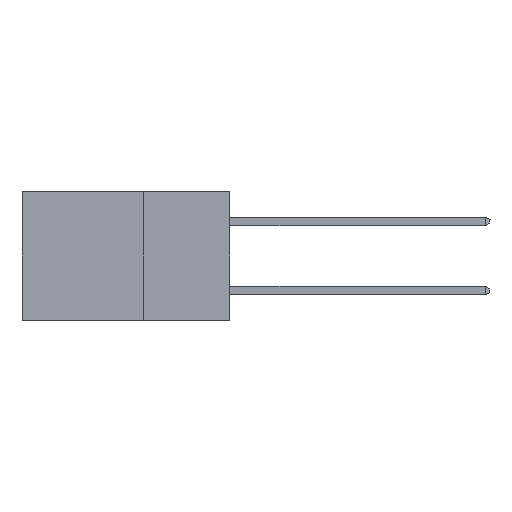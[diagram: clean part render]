
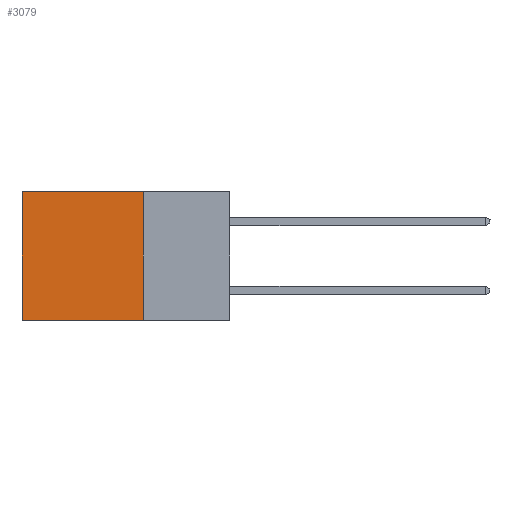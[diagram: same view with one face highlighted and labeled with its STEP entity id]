
A CAD part, left-side view. The second image highlights one B-rep face of the part: STEP entity #3079.
In plain terms, the highlighted planar face has unit normal (-1, 0, 0).
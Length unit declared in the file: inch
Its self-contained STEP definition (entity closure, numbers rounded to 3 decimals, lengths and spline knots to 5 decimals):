
#244 = DIRECTION ( 'NONE',  ( 0., 1., 0. ) ) ;
#1169 = ORIENTED_EDGE ( 'NONE', *, *, #16890, .F. ) ;
#1920 = VECTOR ( 'NONE', #7030, 39.37008 ) ;
#2679 = ORIENTED_EDGE ( 'NONE', *, *, #18009, .T. ) ;
#3079 = ADVANCED_FACE ( 'NONE', ( #25911 ), #11441, .F. ) ;
#3722 = CARTESIAN_POINT ( 'NONE',  ( 0.298, 0.6, -0.37 ) ) ;
#4624 = CARTESIAN_POINT ( 'NONE',  ( 0.298, 0.6, 0. ) ) ;
#5027 = CARTESIAN_POINT ( 'NONE',  ( 0.298, 0.25, 0. ) ) ;
#6023 = DIRECTION ( 'NONE',  ( 0., 0., -1. ) ) ;
#6082 = EDGE_CURVE ( 'NONE', #16232, #9276, #14364, .T. ) ;
#6126 = LINE ( 'NONE', #19397, #12522 ) ;
#6739 = CARTESIAN_POINT ( 'NONE',  ( 0.298, 0.25, 0. ) ) ;
#6807 = CARTESIAN_POINT ( 'NONE',  ( 0.298, 0.25, 0. ) ) ;
#6871 = CARTESIAN_POINT ( 'NONE',  ( 0.298, 0.6, 0. ) ) ;
#7030 = DIRECTION ( 'NONE',  ( 0., 0., -1. ) ) ;
#9276 = VERTEX_POINT ( 'NONE', #6871 ) ;
#9402 = VECTOR ( 'NONE', #6023, 39.37008 ) ;
#11441 = PLANE ( 'NONE',  #20034 ) ;
#11547 = DIRECTION ( 'NONE',  ( 0., 0., -1. ) ) ;
#11553 = VERTEX_POINT ( 'NONE', #19259 ) ;
#11822 = VERTEX_POINT ( 'NONE', #3722 ) ;
#12348 = EDGE_CURVE ( 'NONE', #16232, #11553, #15816, .T. ) ;
#12522 = VECTOR ( 'NONE', #244, 39.37008 ) ;
#14364 = LINE ( 'NONE', #6739, #27091 ) ;
#15816 = LINE ( 'NONE', #29953, #9402 ) ;
#16232 = VERTEX_POINT ( 'NONE', #5027 ) ;
#16890 = EDGE_CURVE ( 'NONE', #11553, #11822, #6126, .T. ) ;
#18009 = EDGE_CURVE ( 'NONE', #9276, #11822, #21054, .T. ) ;
#19259 = CARTESIAN_POINT ( 'NONE',  ( 0.298, 0.25, -0.37 ) ) ;
#19339 = ORIENTED_EDGE ( 'NONE', *, *, #6082, .T. ) ;
#19397 = CARTESIAN_POINT ( 'NONE',  ( 0.298, 0.25, -0.37 ) ) ;
#19933 = ORIENTED_EDGE ( 'NONE', *, *, #12348, .F. ) ;
#20034 = AXIS2_PLACEMENT_3D ( 'NONE', #6807, #21838, #11547 ) ;
#21054 = LINE ( 'NONE', #4624, #1920 ) ;
#21838 = DIRECTION ( 'NONE',  ( 1., 0., 0. ) ) ;
#23532 = DIRECTION ( 'NONE',  ( 0., 1., 0. ) ) ;
#25911 = FACE_OUTER_BOUND ( 'NONE', #28702, .T. ) ;
#27091 = VECTOR ( 'NONE', #23532, 39.37008 ) ;
#28702 = EDGE_LOOP ( 'NONE', ( #2679, #1169, #19933, #19339 ) ) ;
#29953 = CARTESIAN_POINT ( 'NONE',  ( 0.298, 0.25, 0. ) ) ;
